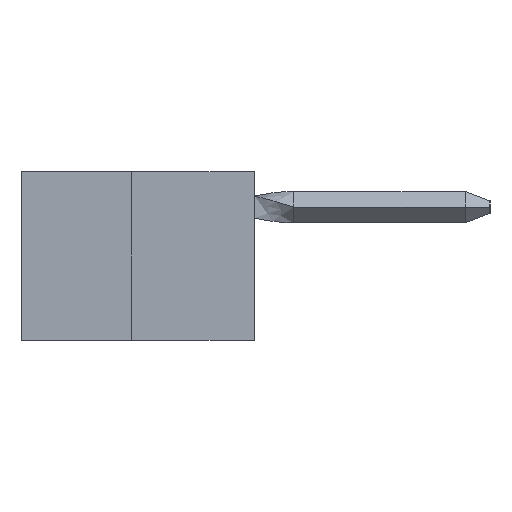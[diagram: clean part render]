
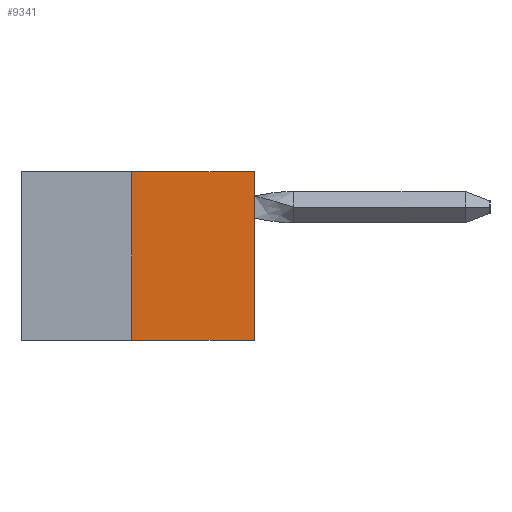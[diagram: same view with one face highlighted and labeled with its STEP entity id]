
A CAD part, left-side view. The second image highlights one B-rep face of the part: STEP entity #9341.
In plain terms, the highlighted planar face has unit normal (-1, 0, 0).
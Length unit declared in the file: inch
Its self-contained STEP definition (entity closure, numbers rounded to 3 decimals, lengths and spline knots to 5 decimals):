
#79 = VERTEX_POINT ( 'NONE', #17572 ) ;
#745 = LINE ( 'NONE', #18475, #18763 ) ;
#1439 = CARTESIAN_POINT ( 'NONE',  ( 0., 0., -0.343 ) ) ;
#1844 = CARTESIAN_POINT ( 'NONE',  ( 0., 0.25, 0. ) ) ;
#2180 = EDGE_CURVE ( 'NONE', #15178, #79, #745, .T. ) ;
#2485 = DIRECTION ( 'NONE',  ( 0., 0., -1. ) ) ;
#4220 = LINE ( 'NONE', #6461, #12259 ) ;
#4741 = DIRECTION ( 'NONE',  ( 0., 0., 1. ) ) ;
#5678 = EDGE_CURVE ( 'NONE', #20962, #79, #11743, .T. ) ;
#6307 = DIRECTION ( 'NONE',  ( 0., 0., 1. ) ) ;
#6440 = EDGE_CURVE ( 'NONE', #7260, #15178, #4220, .T. ) ;
#6461 = CARTESIAN_POINT ( 'NONE',  ( 0., 0.25, 0. ) ) ;
#7034 = VECTOR ( 'NONE', #4741, 39.37008 ) ;
#7260 = VERTEX_POINT ( 'NONE', #17279 ) ;
#9341 = ADVANCED_FACE ( 'NONE', ( #17863 ), #11619, .F. ) ;
#9677 = DIRECTION ( 'NONE',  ( 1., 0., 0. ) ) ;
#11619 = PLANE ( 'NONE',  #14237 ) ;
#11743 = LINE ( 'NONE', #20676, #7034 ) ;
#11779 = DIRECTION ( 'NONE',  ( 0., -1., 0. ) ) ;
#12013 = CARTESIAN_POINT ( 'NONE',  ( 0., 0.473, -0.343 ) ) ;
#12259 = VECTOR ( 'NONE', #6307, 39.37008 ) ;
#12877 = ORIENTED_EDGE ( 'NONE', *, *, #5678, .T. ) ;
#13414 = ORIENTED_EDGE ( 'NONE', *, *, #6440, .F. ) ;
#14237 = AXIS2_PLACEMENT_3D ( 'NONE', #18647, #9677, #2485 ) ;
#15178 = VERTEX_POINT ( 'NONE', #1844 ) ;
#15244 = EDGE_LOOP ( 'NONE', ( #20650, #13414, #18361, #12877 ) ) ;
#16819 = VECTOR ( 'NONE', #11779, 39.37008 ) ;
#17279 = CARTESIAN_POINT ( 'NONE',  ( 0., 0.25, -0.343 ) ) ;
#17439 = EDGE_CURVE ( 'NONE', #7260, #20962, #22955, .T. ) ;
#17572 = CARTESIAN_POINT ( 'NONE',  ( 0., 0., 0. ) ) ;
#17863 = FACE_OUTER_BOUND ( 'NONE', #15244, .T. ) ;
#18361 = ORIENTED_EDGE ( 'NONE', *, *, #17439, .T. ) ;
#18475 = CARTESIAN_POINT ( 'NONE',  ( 0., 0.473, 0. ) ) ;
#18647 = CARTESIAN_POINT ( 'NONE',  ( 0., 0.473, 0. ) ) ;
#18763 = VECTOR ( 'NONE', #20033, 39.37008 ) ;
#20033 = DIRECTION ( 'NONE',  ( 0., -1., 0. ) ) ;
#20650 = ORIENTED_EDGE ( 'NONE', *, *, #2180, .F. ) ;
#20676 = CARTESIAN_POINT ( 'NONE',  ( 0., 0., 0. ) ) ;
#20962 = VERTEX_POINT ( 'NONE', #1439 ) ;
#22955 = LINE ( 'NONE', #12013, #16819 ) ;
